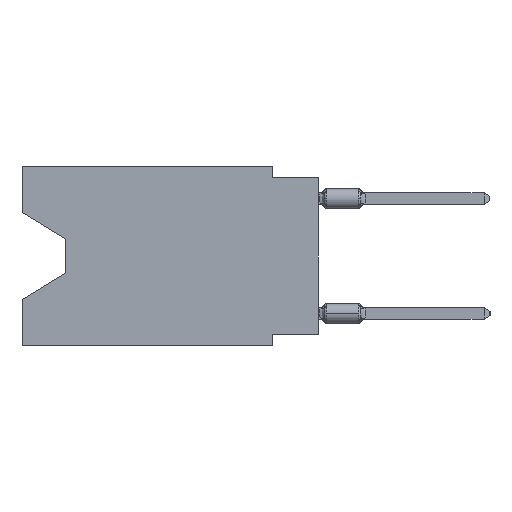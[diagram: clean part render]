
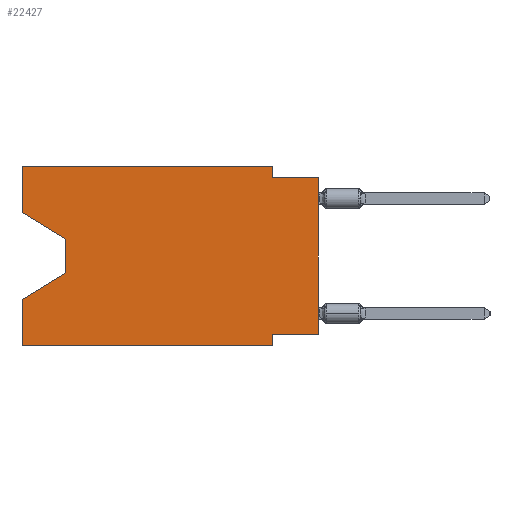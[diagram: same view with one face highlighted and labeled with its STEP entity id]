
A CAD part, left-side view. The second image highlights one B-rep face of the part: STEP entity #22427.
In plain terms, the highlighted planar face has unit normal (-1, 0, 0).
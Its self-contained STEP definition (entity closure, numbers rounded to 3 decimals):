
#192 = EDGE_CURVE ( 'NONE', #18576, #24413, #13808, .T. ) ;
#405 = LINE ( 'NONE', #4861, #12794 ) ;
#1528 = LINE ( 'NONE', #25645, #10389 ) ;
#1871 = FACE_OUTER_BOUND ( 'NONE', #24895, .T. ) ;
#2145 = DIRECTION ( 'NONE',  ( 1., 0., 0. ) ) ;
#2285 = ORIENTED_EDGE ( 'NONE', *, *, #16686, .T. ) ;
#2439 = VERTEX_POINT ( 'NONE', #24717 ) ;
#2464 = LINE ( 'NONE', #4641, #8268 ) ;
#2610 = CARTESIAN_POINT ( 'NONE',  ( 0., 13.97, -5.893 ) ) ;
#2709 = ORIENTED_EDGE ( 'NONE', *, *, #9303, .F. ) ;
#2883 = CARTESIAN_POINT ( 'NONE',  ( 0., 0., -0.635 ) ) ;
#3817 = CARTESIAN_POINT ( 'NONE',  ( 0., 0., -9.271 ) ) ;
#3834 = DIRECTION ( 'NONE',  ( 0., 0., 1. ) ) ;
#4125 = CARTESIAN_POINT ( 'NONE',  ( 0., 0., 0. ) ) ;
#4263 = CARTESIAN_POINT ( 'NONE',  ( 0., 2.54, -9.906 ) ) ;
#4282 = VECTOR ( 'NONE', #26718, 1000. ) ;
#4312 = VECTOR ( 'NONE', #21390, 1000. ) ;
#4641 = CARTESIAN_POINT ( 'NONE',  ( 0., 16.383, 0. ) ) ;
#4678 = VERTEX_POINT ( 'NONE', #23947 ) ;
#4861 = CARTESIAN_POINT ( 'NONE',  ( 0., 13.97, -4.013 ) ) ;
#4893 = DIRECTION ( 'NONE',  ( 0., 0., -1. ) ) ;
#4917 = EDGE_CURVE ( 'NONE', #5259, #24413, #25917, .T. ) ;
#5062 = VERTEX_POINT ( 'NONE', #4263 ) ;
#5259 = VERTEX_POINT ( 'NONE', #14305 ) ;
#5468 = LINE ( 'NONE', #26702, #26543 ) ;
#5507 = VECTOR ( 'NONE', #26848, 1000. ) ;
#5679 = LINE ( 'NONE', #19024, #7324 ) ;
#6203 = CARTESIAN_POINT ( 'NONE',  ( 0., 16.383, -2.546 ) ) ;
#6564 = ORIENTED_EDGE ( 'NONE', *, *, #23743, .F. ) ;
#7220 = CARTESIAN_POINT ( 'NONE',  ( 0., 16.383, 0. ) ) ;
#7324 = VECTOR ( 'NONE', #25173, 1000. ) ;
#7612 = VERTEX_POINT ( 'NONE', #2610 ) ;
#8166 = VERTEX_POINT ( 'NONE', #10073 ) ;
#8268 = VECTOR ( 'NONE', #22269, 1000. ) ;
#8342 = VERTEX_POINT ( 'NONE', #11859 ) ;
#8538 = EDGE_CURVE ( 'NONE', #4678, #8166, #5679, .T. ) ;
#9074 = CARTESIAN_POINT ( 'NONE',  ( 0., 13.97, -5.893 ) ) ;
#9303 = EDGE_CURVE ( 'NONE', #2439, #11224, #26710, .T. ) ;
#9353 = VERTEX_POINT ( 'NONE', #26991 ) ;
#10073 = CARTESIAN_POINT ( 'NONE',  ( 0., 16.383, -7.36 ) ) ;
#10389 = VECTOR ( 'NONE', #19350, 1000. ) ;
#10666 = ORIENTED_EDGE ( 'NONE', *, *, #8538, .F. ) ;
#10917 = VERTEX_POINT ( 'NONE', #26443 ) ;
#11191 = ORIENTED_EDGE ( 'NONE', *, *, #23677, .T. ) ;
#11224 = VERTEX_POINT ( 'NONE', #25846 ) ;
#11486 = ORIENTED_EDGE ( 'NONE', *, *, #14716, .F. ) ;
#11859 = CARTESIAN_POINT ( 'NONE',  ( 0., 2.54, -9.271 ) ) ;
#12043 = ORIENTED_EDGE ( 'NONE', *, *, #17503, .F. ) ;
#12246 = AXIS2_PLACEMENT_3D ( 'NONE', #13068, #2145, #12937 ) ;
#12315 = ORIENTED_EDGE ( 'NONE', *, *, #12978, .T. ) ;
#12794 = VECTOR ( 'NONE', #13617, 1000. ) ;
#12937 = DIRECTION ( 'NONE',  ( 0., 0., -1. ) ) ;
#12978 = EDGE_CURVE ( 'NONE', #9353, #7612, #405, .T. ) ;
#13068 = CARTESIAN_POINT ( 'NONE',  ( 0., 16.383, 0. ) ) ;
#13617 = DIRECTION ( 'NONE',  ( 0., 0., -1. ) ) ;
#13808 = LINE ( 'NONE', #2883, #4282 ) ;
#13984 = EDGE_CURVE ( 'NONE', #10917, #2439, #2464, .T. ) ;
#14305 = CARTESIAN_POINT ( 'NONE',  ( 0., 0., -9.271 ) ) ;
#14391 = ORIENTED_EDGE ( 'NONE', *, *, #192, .F. ) ;
#14716 = EDGE_CURVE ( 'NONE', #11224, #18576, #26473, .T. ) ;
#14737 = DIRECTION ( 'NONE',  ( 0., 1., 0. ) ) ;
#15573 = DIRECTION ( 'NONE',  ( 0., 0., -1. ) ) ;
#15675 = VECTOR ( 'NONE', #15573, 1000. ) ;
#16119 = ORIENTED_EDGE ( 'NONE', *, *, #27036, .T. ) ;
#16686 = EDGE_CURVE ( 'NONE', #10917, #9353, #27871, .T. ) ;
#16869 = VECTOR ( 'NONE', #3834, 1000. ) ;
#17230 = LINE ( 'NONE', #9074, #18770 ) ;
#17503 = EDGE_CURVE ( 'NONE', #5259, #8342, #25768, .T. ) ;
#17809 = DIRECTION ( 'NONE',  ( 0., 0.855, -0.519 ) ) ;
#18576 = VERTEX_POINT ( 'NONE', #20694 ) ;
#18770 = VECTOR ( 'NONE', #17809, 1000. ) ;
#18857 = VECTOR ( 'NONE', #14737, 1000. ) ;
#19024 = CARTESIAN_POINT ( 'NONE',  ( 0., 16.383, 0. ) ) ;
#19350 = DIRECTION ( 'NONE',  ( 0., -1., 0. ) ) ;
#20455 = CARTESIAN_POINT ( 'NONE',  ( 0., 2.54, 0. ) ) ;
#20694 = CARTESIAN_POINT ( 'NONE',  ( 0., 2.54, -0.635 ) ) ;
#21390 = DIRECTION ( 'NONE',  ( 0., -0.855, -0.519 ) ) ;
#22269 = DIRECTION ( 'NONE',  ( 0., 0., 1. ) ) ;
#22427 = ADVANCED_FACE ( 'NONE', ( #1871 ), #28278, .F. ) ;
#23677 = EDGE_CURVE ( 'NONE', #7612, #8166, #17230, .T. ) ;
#23743 = EDGE_CURVE ( 'NONE', #8342, #5062, #5468, .T. ) ;
#23836 = ORIENTED_EDGE ( 'NONE', *, *, #13984, .F. ) ;
#23947 = CARTESIAN_POINT ( 'NONE',  ( 0., 16.383, -9.906 ) ) ;
#24413 = VERTEX_POINT ( 'NONE', #28206 ) ;
#24717 = CARTESIAN_POINT ( 'NONE',  ( 0., 16.383, 0. ) ) ;
#24895 = EDGE_LOOP ( 'NONE', ( #2285, #12315, #11191, #10666, #16119, #6564, #12043, #28027, #14391, #11486, #2709, #23836 ) ) ;
#25173 = DIRECTION ( 'NONE',  ( 0., 0., 1. ) ) ;
#25645 = CARTESIAN_POINT ( 'NONE',  ( 0., 16.383, -9.906 ) ) ;
#25768 = LINE ( 'NONE', #3817, #18857 ) ;
#25846 = CARTESIAN_POINT ( 'NONE',  ( 0., 2.54, 0. ) ) ;
#25917 = LINE ( 'NONE', #4125, #16869 ) ;
#26443 = CARTESIAN_POINT ( 'NONE',  ( 0., 16.383, -2.546 ) ) ;
#26473 = LINE ( 'NONE', #20455, #15675 ) ;
#26543 = VECTOR ( 'NONE', #4893, 1000. ) ;
#26702 = CARTESIAN_POINT ( 'NONE',  ( 0., 2.54, -9.906 ) ) ;
#26710 = LINE ( 'NONE', #7220, #5507 ) ;
#26718 = DIRECTION ( 'NONE',  ( 0., -1., 0. ) ) ;
#26848 = DIRECTION ( 'NONE',  ( 0., -1., 0. ) ) ;
#26991 = CARTESIAN_POINT ( 'NONE',  ( 0., 13.97, -4.013 ) ) ;
#27036 = EDGE_CURVE ( 'NONE', #4678, #5062, #1528, .T. ) ;
#27871 = LINE ( 'NONE', #6203, #4312 ) ;
#28027 = ORIENTED_EDGE ( 'NONE', *, *, #4917, .T. ) ;
#28206 = CARTESIAN_POINT ( 'NONE',  ( 0., 0., -0.635 ) ) ;
#28278 = PLANE ( 'NONE',  #12246 ) ;
